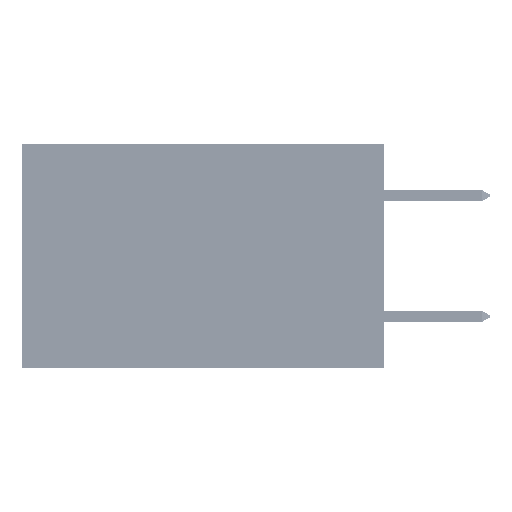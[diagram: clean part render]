
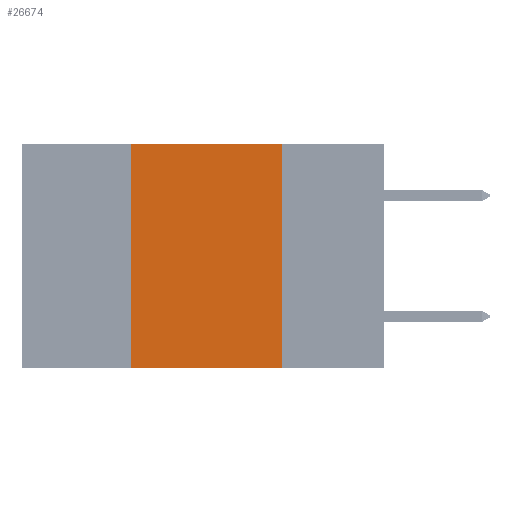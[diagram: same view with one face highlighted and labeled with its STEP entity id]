
A CAD part, left-side view. The second image highlights one B-rep face of the part: STEP entity #26674.
In plain terms, the highlighted planar face has unit normal (-1, 0, 0).
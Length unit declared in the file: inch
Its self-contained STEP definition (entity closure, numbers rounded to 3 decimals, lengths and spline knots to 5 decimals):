
#232 = VECTOR ( 'NONE', #4435, 39.37008 ) ;
#1288 = EDGE_CURVE ( 'NONE', #5318, #34789, #11437, .T. ) ;
#4435 = DIRECTION ( 'NONE',  ( 0., 0., 1. ) ) ;
#4943 = DIRECTION ( 'NONE',  ( 0., -1., 0. ) ) ;
#5318 = VERTEX_POINT ( 'NONE', #29161 ) ;
#6142 = DIRECTION ( 'NONE',  ( 0., -1., 0. ) ) ;
#7944 = PLANE ( 'NONE',  #19418 ) ;
#8188 = FACE_OUTER_BOUND ( 'NONE', #29101, .T. ) ;
#9005 = CARTESIAN_POINT ( 'NONE',  ( 0., 0.6, 0. ) ) ;
#9938 = ORIENTED_EDGE ( 'NONE', *, *, #37831, .F. ) ;
#11437 = LINE ( 'NONE', #15730, #31941 ) ;
#12142 = LINE ( 'NONE', #9005, #35584 ) ;
#13417 = EDGE_CURVE ( 'NONE', #38241, #5318, #12142, .T. ) ;
#15605 = DIRECTION ( 'NONE',  ( 0., 0., -1. ) ) ;
#15730 = CARTESIAN_POINT ( 'NONE',  ( 0., 0.17, 0. ) ) ;
#19080 = VERTEX_POINT ( 'NONE', #40231 ) ;
#19418 = AXIS2_PLACEMENT_3D ( 'NONE', #38093, #22791, #15605 ) ;
#22153 = CARTESIAN_POINT ( 'NONE',  ( 0., 0.42, 0. ) ) ;
#22508 = CARTESIAN_POINT ( 'NONE',  ( 0., 0.42, 0. ) ) ;
#22679 = DIRECTION ( 'NONE',  ( 0., 0., -1. ) ) ;
#22791 = DIRECTION ( 'NONE',  ( 1., 0., 0. ) ) ;
#26674 = ADVANCED_FACE ( 'NONE', ( #8188 ), #7944, .F. ) ;
#29101 = EDGE_LOOP ( 'NONE', ( #39658, #33705, #9938, #43020 ) ) ;
#29161 = CARTESIAN_POINT ( 'NONE',  ( 0., 0.17, 0. ) ) ;
#29362 = VECTOR ( 'NONE', #6142, 39.37008 ) ;
#29577 = LINE ( 'NONE', #22153, #232 ) ;
#31941 = VECTOR ( 'NONE', #22679, 39.37008 ) ;
#32186 = CARTESIAN_POINT ( 'NONE',  ( 0., 0.17, -0.37 ) ) ;
#33705 = ORIENTED_EDGE ( 'NONE', *, *, #13417, .F. ) ;
#34789 = VERTEX_POINT ( 'NONE', #32186 ) ;
#35110 = CARTESIAN_POINT ( 'NONE',  ( 0., 0.6, -0.37 ) ) ;
#35584 = VECTOR ( 'NONE', #4943, 39.37008 ) ;
#37831 = EDGE_CURVE ( 'NONE', #19080, #38241, #29577, .T. ) ;
#38093 = CARTESIAN_POINT ( 'NONE',  ( 0., 0.6, 0. ) ) ;
#38241 = VERTEX_POINT ( 'NONE', #22508 ) ;
#38832 = EDGE_CURVE ( 'NONE', #19080, #34789, #42774, .T. ) ;
#39658 = ORIENTED_EDGE ( 'NONE', *, *, #1288, .F. ) ;
#40231 = CARTESIAN_POINT ( 'NONE',  ( 0., 0.42, -0.37 ) ) ;
#42774 = LINE ( 'NONE', #35110, #29362 ) ;
#43020 = ORIENTED_EDGE ( 'NONE', *, *, #38832, .T. ) ;
